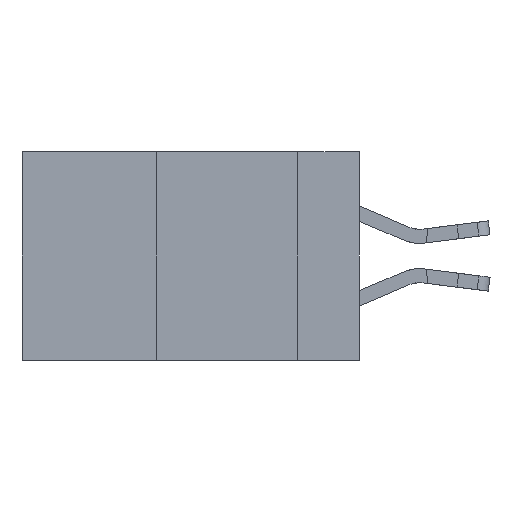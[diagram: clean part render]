
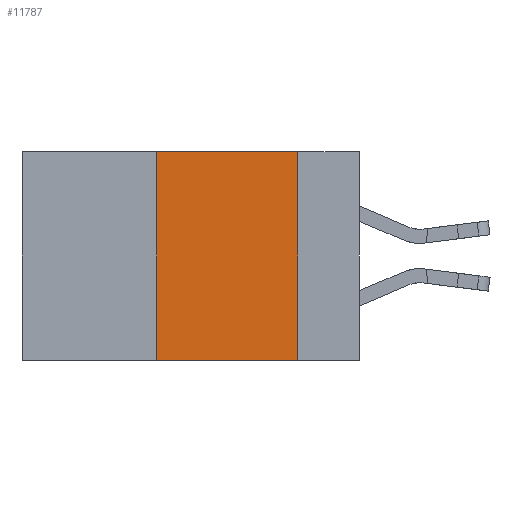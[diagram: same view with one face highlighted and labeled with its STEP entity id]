
A CAD part, left-side view. The second image highlights one B-rep face of the part: STEP entity #11787.
In plain terms, the highlighted planar face has unit normal (-1, 0, 0).
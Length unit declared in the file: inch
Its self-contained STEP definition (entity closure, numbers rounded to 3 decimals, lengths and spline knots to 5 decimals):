
#388 = DIRECTION ( 'NONE',  ( 1., 0., 0. ) ) ;
#1683 = VECTOR ( 'NONE', #12912, 39.37008 ) ;
#1922 = CARTESIAN_POINT ( 'NONE',  ( 0., 0.11, 0. ) ) ;
#2613 = DIRECTION ( 'NONE',  ( 0., -1., 0. ) ) ;
#3621 = VERTEX_POINT ( 'NONE', #12004 ) ;
#3924 = CARTESIAN_POINT ( 'NONE',  ( 0., 0.36, 0. ) ) ;
#4191 = ORIENTED_EDGE ( 'NONE', *, *, #5155, .F. ) ;
#4442 = CARTESIAN_POINT ( 'NONE',  ( 0., 0.6, -0.37 ) ) ;
#5003 = VECTOR ( 'NONE', #2613, 39.37008 ) ;
#5023 = LINE ( 'NONE', #5865, #1683 ) ;
#5155 = EDGE_CURVE ( 'NONE', #3621, #17047, #14217, .T. ) ;
#5300 = VERTEX_POINT ( 'NONE', #3924 ) ;
#5364 = AXIS2_PLACEMENT_3D ( 'NONE', #11705, #388, #10349 ) ;
#5865 = CARTESIAN_POINT ( 'NONE',  ( 0., 0.36, 0. ) ) ;
#6713 = CARTESIAN_POINT ( 'NONE',  ( 0., 0.36, -0.37 ) ) ;
#7335 = DIRECTION ( 'NONE',  ( 0., -1., 0. ) ) ;
#8005 = ORIENTED_EDGE ( 'NONE', *, *, #9920, .T. ) ;
#8030 = EDGE_CURVE ( 'NONE', #10856, #5300, #5023, .T. ) ;
#8491 = EDGE_CURVE ( 'NONE', #5300, #3621, #15858, .T. ) ;
#8726 = FACE_OUTER_BOUND ( 'NONE', #15336, .T. ) ;
#8739 = CARTESIAN_POINT ( 'NONE',  ( 0., 0.11, -0.37 ) ) ;
#8886 = ORIENTED_EDGE ( 'NONE', *, *, #8030, .F. ) ;
#9878 = VECTOR ( 'NONE', #7335, 39.37008 ) ;
#9920 = EDGE_CURVE ( 'NONE', #10856, #17047, #17373, .T. ) ;
#10349 = DIRECTION ( 'NONE',  ( 0., 0., -1. ) ) ;
#10856 = VERTEX_POINT ( 'NONE', #6713 ) ;
#11132 = CARTESIAN_POINT ( 'NONE',  ( 0., 0.6, 0. ) ) ;
#11705 = CARTESIAN_POINT ( 'NONE',  ( 0., 0.6, 0. ) ) ;
#11747 = ORIENTED_EDGE ( 'NONE', *, *, #8491, .F. ) ;
#11787 = ADVANCED_FACE ( 'NONE', ( #8726 ), #17371, .F. ) ;
#12004 = CARTESIAN_POINT ( 'NONE',  ( 0., 0.11, 0. ) ) ;
#12912 = DIRECTION ( 'NONE',  ( 0., 0., 1. ) ) ;
#13314 = DIRECTION ( 'NONE',  ( 0., 0., -1. ) ) ;
#14217 = LINE ( 'NONE', #1922, #17515 ) ;
#15336 = EDGE_LOOP ( 'NONE', ( #4191, #11747, #8886, #8005 ) ) ;
#15858 = LINE ( 'NONE', #11132, #5003 ) ;
#17047 = VERTEX_POINT ( 'NONE', #8739 ) ;
#17371 = PLANE ( 'NONE',  #5364 ) ;
#17373 = LINE ( 'NONE', #4442, #9878 ) ;
#17515 = VECTOR ( 'NONE', #13314, 39.37008 ) ;
